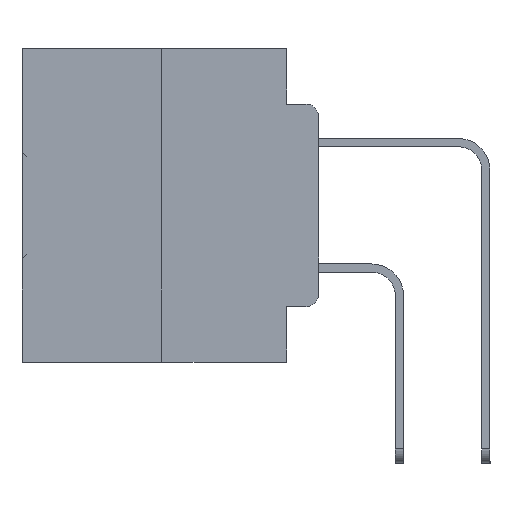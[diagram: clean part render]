
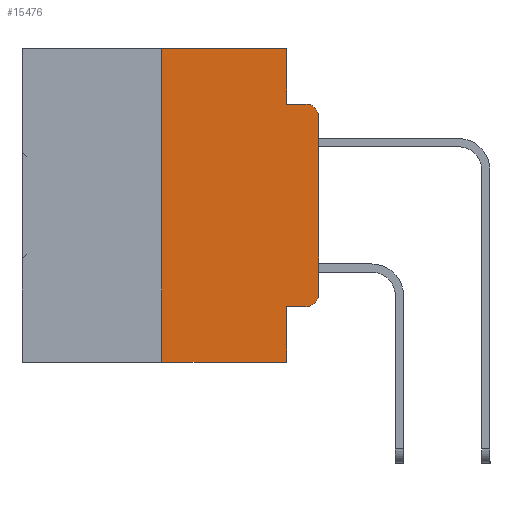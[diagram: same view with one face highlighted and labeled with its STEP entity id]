
A CAD part, left-side view. The second image highlights one B-rep face of the part: STEP entity #15476.
In plain terms, the highlighted planar face has unit normal (-1, 0, 0).
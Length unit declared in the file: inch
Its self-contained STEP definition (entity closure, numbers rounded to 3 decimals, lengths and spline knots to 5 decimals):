
#38 = DIRECTION ( 'NONE',  ( -1., 0., 0. ) ) ;
#546 = ORIENTED_EDGE ( 'NONE', *, *, #4235, .F. ) ;
#1394 = CARTESIAN_POINT ( 'NONE',  ( 0., 0.051, 0. ) ) ;
#1973 = VERTEX_POINT ( 'NONE', #32657 ) ;
#2587 = LINE ( 'NONE', #20568, #31105 ) ;
#2879 = VERTEX_POINT ( 'NONE', #18051 ) ;
#3062 = ORIENTED_EDGE ( 'NONE', *, *, #22155, .T. ) ;
#4063 = EDGE_CURVE ( 'NONE', #22894, #12875, #33785, .T. ) ;
#4235 = EDGE_CURVE ( 'NONE', #21883, #29240, #15914, .T. ) ;
#4503 = EDGE_CURVE ( 'NONE', #1973, #29240, #6257, .T. ) ;
#4707 = EDGE_CURVE ( 'NONE', #16107, #2879, #14120, .T. ) ;
#4802 = AXIS2_PLACEMENT_3D ( 'NONE', #28506, #28627, #12176 ) ;
#5048 = ORIENTED_EDGE ( 'NONE', *, *, #4063, .T. ) ;
#5144 = CARTESIAN_POINT ( 'NONE',  ( 0., 0.02, -0.0885 ) ) ;
#5304 = EDGE_CURVE ( 'NONE', #16107, #13760, #10567, .T. ) ;
#6151 = CARTESIAN_POINT ( 'NONE',  ( 0., 0.051, -0.4115 ) ) ;
#6257 = CIRCLE ( 'NONE', #19943, 0.02 ) ;
#7278 = VECTOR ( 'NONE', #15675, 39.37008 ) ;
#7598 = CARTESIAN_POINT ( 'NONE',  ( 0., 0.02, -0.3915 ) ) ;
#7669 = CARTESIAN_POINT ( 'NONE',  ( 0., 0.051, 0. ) ) ;
#8150 = CARTESIAN_POINT ( 'NONE',  ( 0., 0.051, -0.4115 ) ) ;
#8961 = DIRECTION ( 'NONE',  ( 0., -1., 0. ) ) ;
#9201 = CARTESIAN_POINT ( 'NONE',  ( 0., 0.051, -0.0885 ) ) ;
#9409 = ORIENTED_EDGE ( 'NONE', *, *, #23993, .F. ) ;
#9544 = DIRECTION ( 'NONE',  ( 0., 0., -1. ) ) ;
#10391 = DIRECTION ( 'NONE',  ( 0., 0., -1. ) ) ;
#10567 = LINE ( 'NONE', #20170, #32417 ) ;
#11380 = CARTESIAN_POINT ( 'NONE',  ( 0., 0., -0.3915 ) ) ;
#11970 = VECTOR ( 'NONE', #8961, 39.37008 ) ;
#12176 = DIRECTION ( 'NONE',  ( 0., 0., -1. ) ) ;
#12229 = DIRECTION ( 'NONE',  ( 0., -1., 0. ) ) ;
#12371 = DIRECTION ( 'NONE',  ( 0., -1., 0. ) ) ;
#12524 = CARTESIAN_POINT ( 'NONE',  ( 0., 0.25, -0.5 ) ) ;
#12862 = CARTESIAN_POINT ( 'NONE',  ( 0., 0.473, 0. ) ) ;
#12875 = VERTEX_POINT ( 'NONE', #28478 ) ;
#13760 = VERTEX_POINT ( 'NONE', #21409 ) ;
#14120 = LINE ( 'NONE', #28665, #20589 ) ;
#14653 = DIRECTION ( 'NONE',  ( 0., 0., 1. ) ) ;
#14804 = EDGE_CURVE ( 'NONE', #35252, #21883, #2587, .T. ) ;
#15240 = CIRCLE ( 'NONE', #35747, 0.02 ) ;
#15476 = ADVANCED_FACE ( 'NONE', ( #30628 ), #25921, .F. ) ;
#15675 = DIRECTION ( 'NONE',  ( 0., -1., 0. ) ) ;
#15914 = LINE ( 'NONE', #31518, #28710 ) ;
#16107 = VERTEX_POINT ( 'NONE', #12524 ) ;
#16756 = EDGE_CURVE ( 'NONE', #22894, #2879, #25035, .T. ) ;
#16788 = ORIENTED_EDGE ( 'NONE', *, *, #21739, .T. ) ;
#16876 = CARTESIAN_POINT ( 'NONE',  ( 0., 0.02, -0.1085 ) ) ;
#18051 = CARTESIAN_POINT ( 'NONE',  ( 0., 0.051, -0.5 ) ) ;
#18509 = ORIENTED_EDGE ( 'NONE', *, *, #4503, .T. ) ;
#19620 = DIRECTION ( 'NONE',  ( 0., 0., -1. ) ) ;
#19943 = AXIS2_PLACEMENT_3D ( 'NONE', #16876, #38, #19620 ) ;
#20170 = CARTESIAN_POINT ( 'NONE',  ( 0., 0.25, 0. ) ) ;
#20568 = CARTESIAN_POINT ( 'NONE',  ( 0., 0.051, 0. ) ) ;
#20589 = VECTOR ( 'NONE', #12229, 39.37008 ) ;
#20835 = LINE ( 'NONE', #35284, #34396 ) ;
#21409 = CARTESIAN_POINT ( 'NONE',  ( 0., 0.25, 0. ) ) ;
#21739 = EDGE_CURVE ( 'NONE', #25584, #1973, #20835, .T. ) ;
#21883 = VERTEX_POINT ( 'NONE', #9201 ) ;
#22005 = LINE ( 'NONE', #12862, #7278 ) ;
#22155 = EDGE_CURVE ( 'NONE', #12875, #25584, #15240, .T. ) ;
#22894 = VERTEX_POINT ( 'NONE', #8150 ) ;
#23993 = EDGE_CURVE ( 'NONE', #13760, #35252, #22005, .T. ) ;
#24339 = EDGE_LOOP ( 'NONE', ( #16788, #18509, #546, #24511, #9409, #32979, #27515, #33418, #5048, #3062 ) ) ;
#24511 = ORIENTED_EDGE ( 'NONE', *, *, #14804, .F. ) ;
#25035 = LINE ( 'NONE', #1394, #31378 ) ;
#25584 = VERTEX_POINT ( 'NONE', #11380 ) ;
#25921 = PLANE ( 'NONE',  #4802 ) ;
#26911 = DIRECTION ( 'NONE',  ( -1., 0., 0. ) ) ;
#27276 = DIRECTION ( 'NONE',  ( 0., 0., 1. ) ) ;
#27515 = ORIENTED_EDGE ( 'NONE', *, *, #4707, .T. ) ;
#28478 = CARTESIAN_POINT ( 'NONE',  ( 0., 0.02, -0.4115 ) ) ;
#28506 = CARTESIAN_POINT ( 'NONE',  ( 0., 0.473, 0. ) ) ;
#28627 = DIRECTION ( 'NONE',  ( 1., 0., 0. ) ) ;
#28665 = CARTESIAN_POINT ( 'NONE',  ( 0., 0.473, -0.5 ) ) ;
#28710 = VECTOR ( 'NONE', #12371, 39.37008 ) ;
#29240 = VERTEX_POINT ( 'NONE', #5144 ) ;
#30628 = FACE_OUTER_BOUND ( 'NONE', #24339, .T. ) ;
#31105 = VECTOR ( 'NONE', #9544, 39.37008 ) ;
#31378 = VECTOR ( 'NONE', #31721, 39.37008 ) ;
#31518 = CARTESIAN_POINT ( 'NONE',  ( 0., 0.051, -0.0885 ) ) ;
#31721 = DIRECTION ( 'NONE',  ( 0., 0., -1. ) ) ;
#32417 = VECTOR ( 'NONE', #14653, 39.37008 ) ;
#32657 = CARTESIAN_POINT ( 'NONE',  ( 0., 0., -0.1085 ) ) ;
#32979 = ORIENTED_EDGE ( 'NONE', *, *, #5304, .F. ) ;
#33418 = ORIENTED_EDGE ( 'NONE', *, *, #16756, .F. ) ;
#33785 = LINE ( 'NONE', #6151, #11970 ) ;
#34396 = VECTOR ( 'NONE', #27276, 39.37008 ) ;
#35252 = VERTEX_POINT ( 'NONE', #7669 ) ;
#35284 = CARTESIAN_POINT ( 'NONE',  ( 0., 0., 0. ) ) ;
#35747 = AXIS2_PLACEMENT_3D ( 'NONE', #7598, #26911, #10391 ) ;
